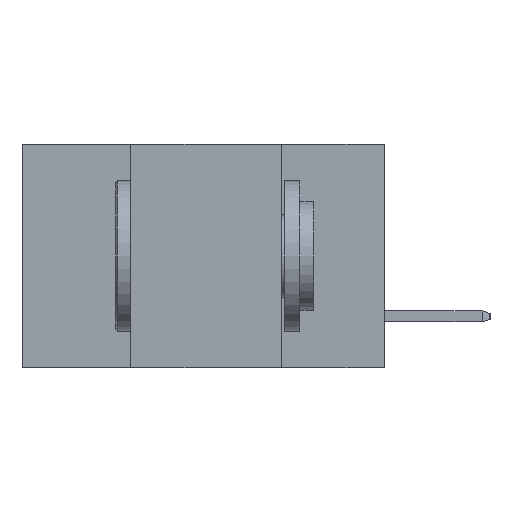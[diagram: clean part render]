
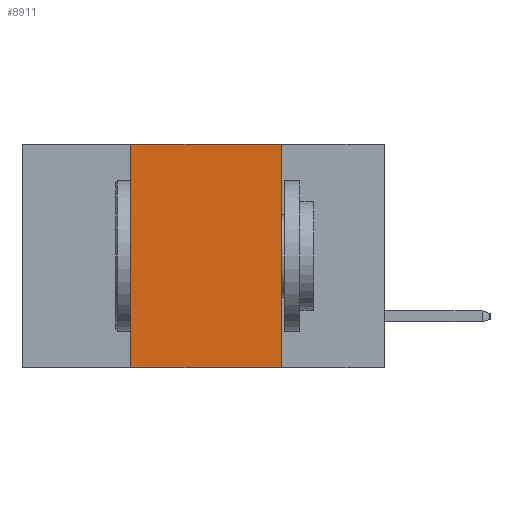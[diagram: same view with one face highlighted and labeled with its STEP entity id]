
A CAD part, left-side view. The second image highlights one B-rep face of the part: STEP entity #8911.
In plain terms, the highlighted planar face has unit normal (-1, 0, 0).
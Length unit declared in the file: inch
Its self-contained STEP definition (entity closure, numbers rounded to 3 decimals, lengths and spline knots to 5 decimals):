
#545 = CARTESIAN_POINT ( 'NONE',  ( 0., 0.42, 0. ) ) ;
#635 = PLANE ( 'NONE',  #18901 ) ;
#730 = VERTEX_POINT ( 'NONE', #17217 ) ;
#947 = VECTOR ( 'NONE', #1484, 39.37008 ) ;
#1484 = DIRECTION ( 'NONE',  ( 0., -1., 0. ) ) ;
#1497 = LINE ( 'NONE', #16280, #947 ) ;
#1592 = CARTESIAN_POINT ( 'NONE',  ( 0., 0.17, 0. ) ) ;
#1599 = EDGE_LOOP ( 'NONE', ( #8457, #13121, #9007, #18197 ) ) ;
#1926 = VERTEX_POINT ( 'NONE', #20710 ) ;
#2422 = DIRECTION ( 'NONE',  ( 0., 0., -1. ) ) ;
#4164 = LINE ( 'NONE', #1592, #4726 ) ;
#4430 = EDGE_CURVE ( 'NONE', #1926, #6039, #4164, .T. ) ;
#4726 = VECTOR ( 'NONE', #16372, 39.37008 ) ;
#6039 = VERTEX_POINT ( 'NONE', #8855 ) ;
#6434 = EDGE_CURVE ( 'NONE', #8528, #6039, #1497, .T. ) ;
#7151 = LINE ( 'NONE', #545, #10706 ) ;
#8457 = ORIENTED_EDGE ( 'NONE', *, *, #4430, .F. ) ;
#8528 = VERTEX_POINT ( 'NONE', #21984 ) ;
#8800 = VECTOR ( 'NONE', #12622, 39.37008 ) ;
#8855 = CARTESIAN_POINT ( 'NONE',  ( 0., 0.17, -0.37 ) ) ;
#8911 = ADVANCED_FACE ( 'NONE', ( #14190 ), #635, .F. ) ;
#9007 = ORIENTED_EDGE ( 'NONE', *, *, #14178, .F. ) ;
#9358 = LINE ( 'NONE', #16112, #8800 ) ;
#10706 = VECTOR ( 'NONE', #14515, 39.37008 ) ;
#11105 = CARTESIAN_POINT ( 'NONE',  ( 0., 0.6, 0. ) ) ;
#12622 = DIRECTION ( 'NONE',  ( 0., -1., 0. ) ) ;
#12859 = DIRECTION ( 'NONE',  ( 1., 0., 0. ) ) ;
#13121 = ORIENTED_EDGE ( 'NONE', *, *, #19284, .F. ) ;
#14178 = EDGE_CURVE ( 'NONE', #8528, #730, #7151, .T. ) ;
#14190 = FACE_OUTER_BOUND ( 'NONE', #1599, .T. ) ;
#14515 = DIRECTION ( 'NONE',  ( 0., 0., 1. ) ) ;
#16112 = CARTESIAN_POINT ( 'NONE',  ( 0., 0.6, 0. ) ) ;
#16280 = CARTESIAN_POINT ( 'NONE',  ( 0., 0.6, -0.37 ) ) ;
#16372 = DIRECTION ( 'NONE',  ( 0., 0., -1. ) ) ;
#17217 = CARTESIAN_POINT ( 'NONE',  ( 0., 0.42, 0. ) ) ;
#18197 = ORIENTED_EDGE ( 'NONE', *, *, #6434, .T. ) ;
#18901 = AXIS2_PLACEMENT_3D ( 'NONE', #11105, #12859, #2422 ) ;
#19284 = EDGE_CURVE ( 'NONE', #730, #1926, #9358, .T. ) ;
#20710 = CARTESIAN_POINT ( 'NONE',  ( 0., 0.17, 0. ) ) ;
#21984 = CARTESIAN_POINT ( 'NONE',  ( 0., 0.42, -0.37 ) ) ;
